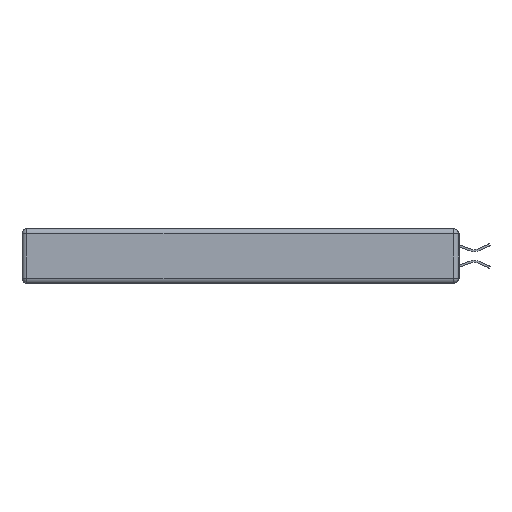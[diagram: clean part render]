
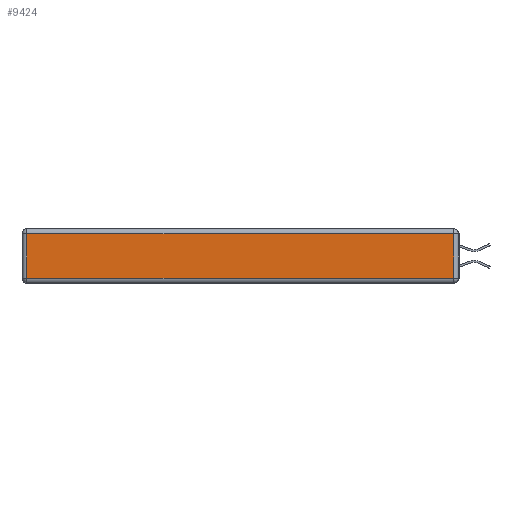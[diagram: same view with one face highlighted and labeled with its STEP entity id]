
A CAD part, left-side view. The second image highlights one B-rep face of the part: STEP entity #9424.
In plain terms, the highlighted planar face has unit normal (-1, 0, 0).
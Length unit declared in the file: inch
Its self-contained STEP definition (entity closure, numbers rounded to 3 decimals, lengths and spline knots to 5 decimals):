
#450 = VECTOR ( 'NONE', #5096, 39.37008 ) ;
#472 = CARTESIAN_POINT ( 'NONE',  ( 0., 2.75, -0.03 ) ) ;
#1084 = CARTESIAN_POINT ( 'NONE',  ( 0., 0., -0.313 ) ) ;
#2301 = ORIENTED_EDGE ( 'NONE', *, *, #16469, .T. ) ;
#3069 = FACE_OUTER_BOUND ( 'NONE', #18394, .T. ) ;
#3178 = PLANE ( 'NONE',  #10965 ) ;
#3801 = LINE ( 'NONE', #1084, #15431 ) ;
#4123 = CARTESIAN_POINT ( 'NONE',  ( 0., 2.72, -0.313 ) ) ;
#4420 = ORIENTED_EDGE ( 'NONE', *, *, #15178, .T. ) ;
#4619 = DIRECTION ( 'NONE',  ( 0., 0., 1. ) ) ;
#5096 = DIRECTION ( 'NONE',  ( 0., 1., 0. ) ) ;
#5475 = ORIENTED_EDGE ( 'NONE', *, *, #11728, .T. ) ;
#6045 = DIRECTION ( 'NONE',  ( 0., 0., -1. ) ) ;
#6899 = LINE ( 'NONE', #13666, #8793 ) ;
#7634 = VERTEX_POINT ( 'NONE', #12580 ) ;
#8667 = VECTOR ( 'NONE', #6045, 39.37008 ) ;
#8793 = VECTOR ( 'NONE', #4619, 39.37008 ) ;
#9135 = EDGE_CURVE ( 'NONE', #12993, #7634, #3801, .T. ) ;
#9424 = ADVANCED_FACE ( 'NONE', ( #3069 ), #3178, .T. ) ;
#10965 = AXIS2_PLACEMENT_3D ( 'NONE', #13773, #16870, #12110 ) ;
#11728 = EDGE_CURVE ( 'NONE', #16387, #12993, #18187, .T. ) ;
#12110 = DIRECTION ( 'NONE',  ( 0., 0., 1. ) ) ;
#12580 = CARTESIAN_POINT ( 'NONE',  ( 0., 0.03, -0.313 ) ) ;
#12993 = VERTEX_POINT ( 'NONE', #4123 ) ;
#13144 = CARTESIAN_POINT ( 'NONE',  ( 0., 0.03, -0.03 ) ) ;
#13666 = CARTESIAN_POINT ( 'NONE',  ( 0., 0.03, -0.343 ) ) ;
#13773 = CARTESIAN_POINT ( 'NONE',  ( 0., 0., -0.343 ) ) ;
#13942 = LINE ( 'NONE', #472, #450 ) ;
#14193 = ORIENTED_EDGE ( 'NONE', *, *, #9135, .T. ) ;
#14787 = DIRECTION ( 'NONE',  ( 0., -1., 0. ) ) ;
#14952 = VERTEX_POINT ( 'NONE', #13144 ) ;
#15062 = CARTESIAN_POINT ( 'NONE',  ( 0., 2.72, -0.343 ) ) ;
#15178 = EDGE_CURVE ( 'NONE', #7634, #14952, #6899, .T. ) ;
#15431 = VECTOR ( 'NONE', #14787, 39.37008 ) ;
#16387 = VERTEX_POINT ( 'NONE', #18376 ) ;
#16469 = EDGE_CURVE ( 'NONE', #14952, #16387, #13942, .T. ) ;
#16870 = DIRECTION ( 'NONE',  ( -1., 0., 0. ) ) ;
#18187 = LINE ( 'NONE', #15062, #8667 ) ;
#18376 = CARTESIAN_POINT ( 'NONE',  ( 0., 2.72, -0.03 ) ) ;
#18394 = EDGE_LOOP ( 'NONE', ( #14193, #4420, #2301, #5475 ) ) ;
